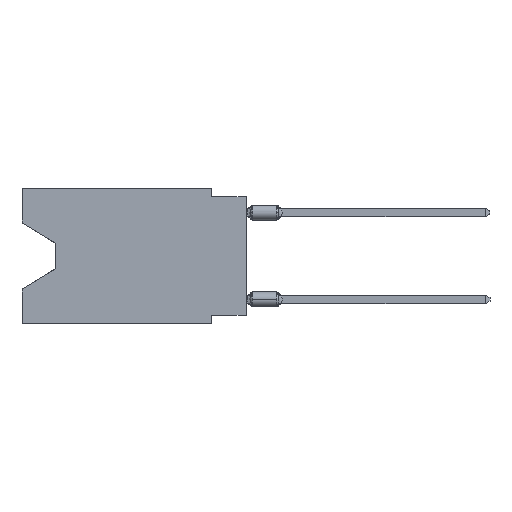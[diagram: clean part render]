
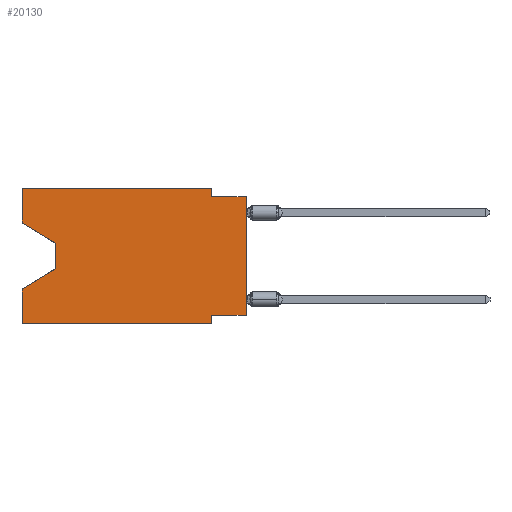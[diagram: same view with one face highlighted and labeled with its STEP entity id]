
A CAD part, left-side view. The second image highlights one B-rep face of the part: STEP entity #20130.
In plain terms, the highlighted planar face has unit normal (-1, 0, 0).
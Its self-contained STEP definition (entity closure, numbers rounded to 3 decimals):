
#176 = ORIENTED_EDGE ( 'NONE', *, *, #9040, .T. ) ;
#206 = DIRECTION ( 'NONE',  ( 0., 1., 0. ) ) ;
#1179 = DIRECTION ( 'NONE',  ( 0., 0., -1. ) ) ;
#1500 = CARTESIAN_POINT ( 'NONE',  ( 0., 16.383, 0. ) ) ;
#1857 = EDGE_CURVE ( 'NONE', #5790, #6759, #29784, .T. ) ;
#2014 = VERTEX_POINT ( 'NONE', #4358 ) ;
#3000 = VECTOR ( 'NONE', #20634, 1000. ) ;
#3036 = VERTEX_POINT ( 'NONE', #21484 ) ;
#4052 = VECTOR ( 'NONE', #9657, 1000. ) ;
#4315 = VECTOR ( 'NONE', #28239, 1000. ) ;
#4358 = CARTESIAN_POINT ( 'NONE',  ( 0., 2.54, -9.906 ) ) ;
#4743 = CARTESIAN_POINT ( 'NONE',  ( 0., 0., -0.635 ) ) ;
#5203 = DIRECTION ( 'NONE',  ( 0., -1., 0. ) ) ;
#5790 = VERTEX_POINT ( 'NONE', #9725 ) ;
#5942 = CARTESIAN_POINT ( 'NONE',  ( 0., 2.54, 0. ) ) ;
#6060 = ORIENTED_EDGE ( 'NONE', *, *, #6848, .T. ) ;
#6163 = EDGE_CURVE ( 'NONE', #23102, #28935, #11913, .T. ) ;
#6574 = DIRECTION ( 'NONE',  ( 0., 0., 1. ) ) ;
#6659 = CARTESIAN_POINT ( 'NONE',  ( 0., 16.383, -9.906 ) ) ;
#6759 = VERTEX_POINT ( 'NONE', #22683 ) ;
#6848 = EDGE_CURVE ( 'NONE', #21563, #28302, #11326, .T. ) ;
#7093 = ORIENTED_EDGE ( 'NONE', *, *, #7878, .F. ) ;
#7134 = CARTESIAN_POINT ( 'NONE',  ( 0., 13.97, -5.893 ) ) ;
#7229 = ORIENTED_EDGE ( 'NONE', *, *, #30128, .F. ) ;
#7328 = CARTESIAN_POINT ( 'NONE',  ( 0., 0., 0. ) ) ;
#7878 = EDGE_CURVE ( 'NONE', #23102, #11686, #17077, .T. ) ;
#8004 = EDGE_CURVE ( 'NONE', #28302, #24656, #9497, .T. ) ;
#8245 = VECTOR ( 'NONE', #11677, 1000. ) ;
#8560 = CARTESIAN_POINT ( 'NONE',  ( 0., 16.383, -2.546 ) ) ;
#8574 = CARTESIAN_POINT ( 'NONE',  ( 0., 16.383, 0. ) ) ;
#8735 = FACE_OUTER_BOUND ( 'NONE', #20621, .T. ) ;
#8973 = LINE ( 'NONE', #18610, #4315 ) ;
#9040 = EDGE_CURVE ( 'NONE', #30839, #21563, #13776, .T. ) ;
#9372 = DIRECTION ( 'NONE',  ( 0., 0., 1. ) ) ;
#9497 = LINE ( 'NONE', #7134, #4052 ) ;
#9655 = CARTESIAN_POINT ( 'NONE',  ( 0., 16.383, 0. ) ) ;
#9657 = DIRECTION ( 'NONE',  ( 0., 0.855, -0.519 ) ) ;
#9725 = CARTESIAN_POINT ( 'NONE',  ( 0., 2.54, 0. ) ) ;
#9727 = EDGE_CURVE ( 'NONE', #30839, #3036, #15853, .T. ) ;
#10602 = VECTOR ( 'NONE', #25306, 1000. ) ;
#11326 = LINE ( 'NONE', #28062, #3000 ) ;
#11677 = DIRECTION ( 'NONE',  ( 0., 0., -1. ) ) ;
#11686 = VERTEX_POINT ( 'NONE', #15481 ) ;
#11913 = LINE ( 'NONE', #7328, #20911 ) ;
#12192 = VECTOR ( 'NONE', #6574, 1000. ) ;
#13490 = DIRECTION ( 'NONE',  ( 0., 0., 1. ) ) ;
#13569 = LINE ( 'NONE', #18621, #8245 ) ;
#13776 = LINE ( 'NONE', #8560, #10602 ) ;
#14406 = LINE ( 'NONE', #9655, #27110 ) ;
#14557 = DIRECTION ( 'NONE',  ( 0., -1., 0. ) ) ;
#15481 = CARTESIAN_POINT ( 'NONE',  ( 0., 2.54, -9.271 ) ) ;
#15687 = DIRECTION ( 'NONE',  ( 1., 0., 0. ) ) ;
#15843 = PLANE ( 'NONE',  #23755 ) ;
#15853 = LINE ( 'NONE', #1500, #23744 ) ;
#16037 = DIRECTION ( 'NONE',  ( 0., 0., -1. ) ) ;
#16419 = VECTOR ( 'NONE', #5203, 1000. ) ;
#16617 = EDGE_CURVE ( 'NONE', #27572, #24656, #25535, .T. ) ;
#17077 = LINE ( 'NONE', #24183, #23674 ) ;
#18398 = CARTESIAN_POINT ( 'NONE',  ( 0., 16.383, -2.546 ) ) ;
#18610 = CARTESIAN_POINT ( 'NONE',  ( 0., 16.383, -9.906 ) ) ;
#18621 = CARTESIAN_POINT ( 'NONE',  ( 0., 2.54, -9.906 ) ) ;
#18916 = ORIENTED_EDGE ( 'NONE', *, *, #1857, .F. ) ;
#19424 = ORIENTED_EDGE ( 'NONE', *, *, #27693, .F. ) ;
#19562 = CARTESIAN_POINT ( 'NONE',  ( 0., 0., -0.635 ) ) ;
#19722 = LINE ( 'NONE', #4743, #16419 ) ;
#19950 = ORIENTED_EDGE ( 'NONE', *, *, #8004, .T. ) ;
#20130 = ADVANCED_FACE ( 'NONE', ( #8735 ), #15843, .F. ) ;
#20621 = EDGE_LOOP ( 'NONE', ( #176, #6060, #19950, #30696, #21130, #20848, #7093, #23435, #7229, #18916, #19424, #24758 ) ) ;
#20634 = DIRECTION ( 'NONE',  ( 0., 0., -1. ) ) ;
#20848 = ORIENTED_EDGE ( 'NONE', *, *, #23201, .F. ) ;
#20911 = VECTOR ( 'NONE', #9372, 1000. ) ;
#20971 = VECTOR ( 'NONE', #16037, 1000. ) ;
#21130 = ORIENTED_EDGE ( 'NONE', *, *, #25193, .T. ) ;
#21484 = CARTESIAN_POINT ( 'NONE',  ( 0., 16.383, 0. ) ) ;
#21563 = VERTEX_POINT ( 'NONE', #25759 ) ;
#22683 = CARTESIAN_POINT ( 'NONE',  ( 0., 2.54, -0.635 ) ) ;
#22993 = CARTESIAN_POINT ( 'NONE',  ( 0., 16.383, 0. ) ) ;
#23102 = VERTEX_POINT ( 'NONE', #30003 ) ;
#23201 = EDGE_CURVE ( 'NONE', #11686, #2014, #13569, .T. ) ;
#23435 = ORIENTED_EDGE ( 'NONE', *, *, #6163, .T. ) ;
#23674 = VECTOR ( 'NONE', #206, 1000. ) ;
#23744 = VECTOR ( 'NONE', #13490, 1000. ) ;
#23755 = AXIS2_PLACEMENT_3D ( 'NONE', #8574, #15687, #1179 ) ;
#24183 = CARTESIAN_POINT ( 'NONE',  ( 0., 0., -9.271 ) ) ;
#24656 = VERTEX_POINT ( 'NONE', #27129 ) ;
#24758 = ORIENTED_EDGE ( 'NONE', *, *, #9727, .F. ) ;
#25193 = EDGE_CURVE ( 'NONE', #27572, #2014, #8973, .T. ) ;
#25306 = DIRECTION ( 'NONE',  ( 0., -0.855, -0.519 ) ) ;
#25535 = LINE ( 'NONE', #22993, #12192 ) ;
#25759 = CARTESIAN_POINT ( 'NONE',  ( 0., 13.97, -4.013 ) ) ;
#27110 = VECTOR ( 'NONE', #14557, 1000. ) ;
#27129 = CARTESIAN_POINT ( 'NONE',  ( 0., 16.383, -7.36 ) ) ;
#27572 = VERTEX_POINT ( 'NONE', #6659 ) ;
#27693 = EDGE_CURVE ( 'NONE', #3036, #5790, #14406, .T. ) ;
#28062 = CARTESIAN_POINT ( 'NONE',  ( 0., 13.97, -4.013 ) ) ;
#28069 = CARTESIAN_POINT ( 'NONE',  ( 0., 13.97, -5.893 ) ) ;
#28239 = DIRECTION ( 'NONE',  ( 0., -1., 0. ) ) ;
#28302 = VERTEX_POINT ( 'NONE', #28069 ) ;
#28935 = VERTEX_POINT ( 'NONE', #19562 ) ;
#29784 = LINE ( 'NONE', #5942, #20971 ) ;
#30003 = CARTESIAN_POINT ( 'NONE',  ( 0., 0., -9.271 ) ) ;
#30128 = EDGE_CURVE ( 'NONE', #6759, #28935, #19722, .T. ) ;
#30696 = ORIENTED_EDGE ( 'NONE', *, *, #16617, .F. ) ;
#30839 = VERTEX_POINT ( 'NONE', #18398 ) ;
